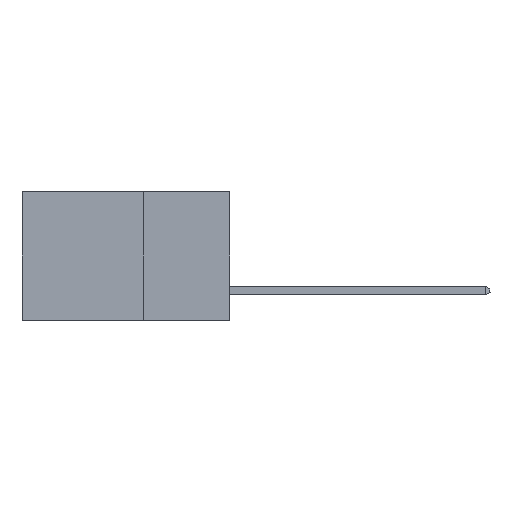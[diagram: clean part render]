
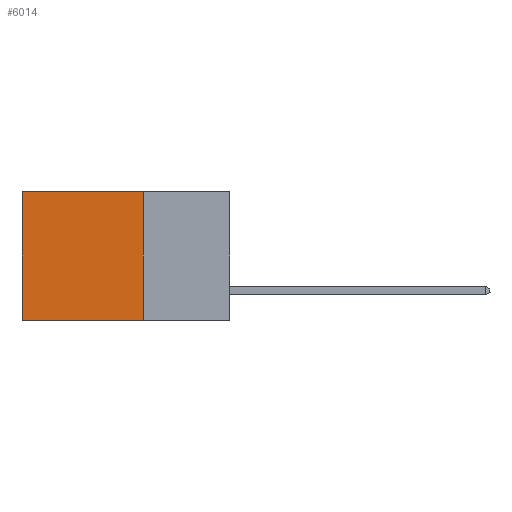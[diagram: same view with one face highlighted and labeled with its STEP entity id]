
A CAD part, left-side view. The second image highlights one B-rep face of the part: STEP entity #6014.
In plain terms, the highlighted planar face has unit normal (-1, 0, 0).
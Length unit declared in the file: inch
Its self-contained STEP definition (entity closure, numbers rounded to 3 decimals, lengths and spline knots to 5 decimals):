
#380 = DIRECTION ( 'NONE',  ( 0., 0., -1. ) ) ;
#691 = VECTOR ( 'NONE', #26737, 39.37008 ) ;
#2261 = EDGE_LOOP ( 'NONE', ( #6334, #10756, #17511, #12995 ) ) ;
#3138 = CARTESIAN_POINT ( 'NONE',  ( 0.298, 0.25, -0.37 ) ) ;
#3372 = EDGE_CURVE ( 'NONE', #3707, #11598, #21963, .T. ) ;
#3707 = VERTEX_POINT ( 'NONE', #5222 ) ;
#4071 = CARTESIAN_POINT ( 'NONE',  ( 0.298, 0.25, 0. ) ) ;
#5222 = CARTESIAN_POINT ( 'NONE',  ( 0.298, 0.25, -0.37 ) ) ;
#5599 = EDGE_CURVE ( 'NONE', #21843, #3707, #24938, .T. ) ;
#6014 = ADVANCED_FACE ( 'NONE', ( #14587 ), #15870, .F. ) ;
#6334 = ORIENTED_EDGE ( 'NONE', *, *, #27552, .T. ) ;
#6454 = DIRECTION ( 'NONE',  ( 1., 0., 0. ) ) ;
#7005 = LINE ( 'NONE', #7715, #691 ) ;
#7438 = CARTESIAN_POINT ( 'NONE',  ( 0.298, 0.6, 0. ) ) ;
#7715 = CARTESIAN_POINT ( 'NONE',  ( 0.298, 0.25, 0. ) ) ;
#9443 = CARTESIAN_POINT ( 'NONE',  ( 0.298, 0.25, 0. ) ) ;
#10756 = ORIENTED_EDGE ( 'NONE', *, *, #3372, .F. ) ;
#11598 = VERTEX_POINT ( 'NONE', #13807 ) ;
#12394 = VECTOR ( 'NONE', #15203, 39.37008 ) ;
#12643 = EDGE_CURVE ( 'NONE', #21843, #21255, #7005, .T. ) ;
#12995 = ORIENTED_EDGE ( 'NONE', *, *, #12643, .T. ) ;
#13521 = CARTESIAN_POINT ( 'NONE',  ( 0.298, 0.6, 0. ) ) ;
#13807 = CARTESIAN_POINT ( 'NONE',  ( 0.298, 0.6, -0.37 ) ) ;
#14587 = FACE_OUTER_BOUND ( 'NONE', #2261, .T. ) ;
#15203 = DIRECTION ( 'NONE',  ( 0., 0., -1. ) ) ;
#15724 = AXIS2_PLACEMENT_3D ( 'NONE', #4071, #6454, #23008 ) ;
#15870 = PLANE ( 'NONE',  #15724 ) ;
#17511 = ORIENTED_EDGE ( 'NONE', *, *, #5599, .F. ) ;
#21236 = LINE ( 'NONE', #7438, #26468 ) ;
#21255 = VERTEX_POINT ( 'NONE', #13521 ) ;
#21843 = VERTEX_POINT ( 'NONE', #9443 ) ;
#21963 = LINE ( 'NONE', #3138, #23103 ) ;
#22331 = CARTESIAN_POINT ( 'NONE',  ( 0.298, 0.25, 0. ) ) ;
#23008 = DIRECTION ( 'NONE',  ( 0., 0., -1. ) ) ;
#23103 = VECTOR ( 'NONE', #27026, 39.37008 ) ;
#24938 = LINE ( 'NONE', #22331, #12394 ) ;
#26468 = VECTOR ( 'NONE', #380, 39.37008 ) ;
#26737 = DIRECTION ( 'NONE',  ( 0., 1., 0. ) ) ;
#27026 = DIRECTION ( 'NONE',  ( 0., 1., 0. ) ) ;
#27552 = EDGE_CURVE ( 'NONE', #21255, #11598, #21236, .T. ) ;
